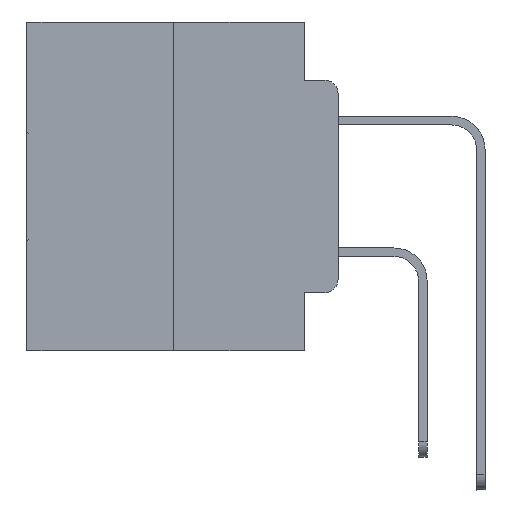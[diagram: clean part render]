
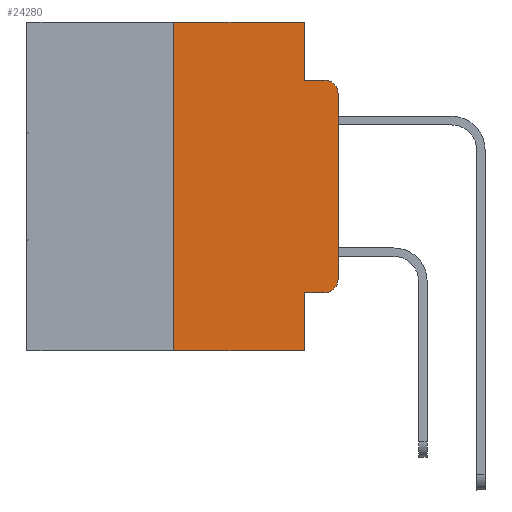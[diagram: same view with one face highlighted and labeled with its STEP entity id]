
A CAD part, left-side view. The second image highlights one B-rep face of the part: STEP entity #24280.
In plain terms, the highlighted planar face has unit normal (-1, 0, 0).
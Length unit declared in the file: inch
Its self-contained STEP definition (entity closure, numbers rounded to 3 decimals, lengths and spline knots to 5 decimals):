
#653 = EDGE_CURVE ( 'NONE', #25237, #11357, #2245, .T. ) ;
#929 = CARTESIAN_POINT ( 'NONE',  ( 0., 0.051, 0. ) ) ;
#1689 = VERTEX_POINT ( 'NONE', #3269 ) ;
#2054 = LINE ( 'NONE', #929, #7876 ) ;
#2245 = LINE ( 'NONE', #30359, #20890 ) ;
#2469 = VECTOR ( 'NONE', #9802, 39.37008 ) ;
#2824 = EDGE_CURVE ( 'NONE', #22098, #25548, #9690, .T. ) ;
#3015 = CARTESIAN_POINT ( 'NONE',  ( 0., 0., -0.3915 ) ) ;
#3049 = CARTESIAN_POINT ( 'NONE',  ( 0., 0., 0. ) ) ;
#3269 = CARTESIAN_POINT ( 'NONE',  ( 0., 0.02, -0.0885 ) ) ;
#3486 = DIRECTION ( 'NONE',  ( 0., 0., -1. ) ) ;
#3506 = AXIS2_PLACEMENT_3D ( 'NONE', #13708, #28260, #13824 ) ;
#3591 = CARTESIAN_POINT ( 'NONE',  ( 0., 0.25, 0. ) ) ;
#3608 = ORIENTED_EDGE ( 'NONE', *, *, #12410, .T. ) ;
#4257 = CARTESIAN_POINT ( 'NONE',  ( 0., 0.02, -0.1085 ) ) ;
#4287 = VERTEX_POINT ( 'NONE', #7870 ) ;
#4773 = VECTOR ( 'NONE', #27959, 39.37008 ) ;
#4962 = EDGE_LOOP ( 'NONE', ( #18984, #26924, #22753, #6592, #11934, #27152, #8615, #22231, #3608, #29385 ) ) ;
#6106 = DIRECTION ( 'NONE',  ( 0., 0., 1. ) ) ;
#6131 = VERTEX_POINT ( 'NONE', #3015 ) ;
#6236 = CARTESIAN_POINT ( 'NONE',  ( 0., 0.051, -0.0885 ) ) ;
#6496 = PLANE ( 'NONE',  #3506 ) ;
#6554 = FACE_OUTER_BOUND ( 'NONE', #4962, .T. ) ;
#6592 = ORIENTED_EDGE ( 'NONE', *, *, #20519, .F. ) ;
#6742 = DIRECTION ( 'NONE',  ( 0., 0., -1. ) ) ;
#7367 = CARTESIAN_POINT ( 'NONE',  ( 0., 0.051, 0. ) ) ;
#7427 = VECTOR ( 'NONE', #26977, 39.37008 ) ;
#7870 = CARTESIAN_POINT ( 'NONE',  ( 0., 0.051, -0.4115 ) ) ;
#7876 = VECTOR ( 'NONE', #3486, 39.37008 ) ;
#8458 = DIRECTION ( 'NONE',  ( -1., 0., 0. ) ) ;
#8495 = CARTESIAN_POINT ( 'NONE',  ( 0., 0., -0.1085 ) ) ;
#8614 = CARTESIAN_POINT ( 'NONE',  ( 0., 0.051, -0.0885 ) ) ;
#8615 = ORIENTED_EDGE ( 'NONE', *, *, #653, .T. ) ;
#9690 = LINE ( 'NONE', #19815, #21775 ) ;
#9732 = CARTESIAN_POINT ( 'NONE',  ( 0., 0.25, 0. ) ) ;
#9802 = DIRECTION ( 'NONE',  ( 0., 0., -1. ) ) ;
#10788 = EDGE_CURVE ( 'NONE', #22335, #6131, #20766, .T. ) ;
#11357 = VERTEX_POINT ( 'NONE', #15563 ) ;
#11416 = LINE ( 'NONE', #3049, #17154 ) ;
#11619 = LINE ( 'NONE', #7367, #2469 ) ;
#11934 = ORIENTED_EDGE ( 'NONE', *, *, #2824, .F. ) ;
#12024 = VERTEX_POINT ( 'NONE', #8495 ) ;
#12410 = EDGE_CURVE ( 'NONE', #4287, #22335, #13913, .T. ) ;
#13522 = VERTEX_POINT ( 'NONE', #6236 ) ;
#13708 = CARTESIAN_POINT ( 'NONE',  ( 0., 0.473, 0. ) ) ;
#13824 = DIRECTION ( 'NONE',  ( 0., 0., -1. ) ) ;
#13830 = CARTESIAN_POINT ( 'NONE',  ( 0., 0.25, -0.5 ) ) ;
#13913 = LINE ( 'NONE', #19788, #7427 ) ;
#14087 = AXIS2_PLACEMENT_3D ( 'NONE', #4257, #21222, #6742 ) ;
#15563 = CARTESIAN_POINT ( 'NONE',  ( 0., 0.051, -0.5 ) ) ;
#16010 = AXIS2_PLACEMENT_3D ( 'NONE', #22927, #8458, #25363 ) ;
#17154 = VECTOR ( 'NONE', #20070, 39.37008 ) ;
#17351 = EDGE_CURVE ( 'NONE', #4287, #11357, #11619, .T. ) ;
#18924 = EDGE_CURVE ( 'NONE', #25237, #22098, #21381, .T. ) ;
#18984 = ORIENTED_EDGE ( 'NONE', *, *, #30165, .T. ) ;
#19788 = CARTESIAN_POINT ( 'NONE',  ( 0., 0.051, -0.4115 ) ) ;
#19815 = CARTESIAN_POINT ( 'NONE',  ( 0., 0.473, 0. ) ) ;
#19908 = DIRECTION ( 'NONE',  ( 0., -1., 0. ) ) ;
#20070 = DIRECTION ( 'NONE',  ( 0., 0., 1. ) ) ;
#20519 = EDGE_CURVE ( 'NONE', #25548, #13522, #2054, .T. ) ;
#20525 = DIRECTION ( 'NONE',  ( 0., -1., 0. ) ) ;
#20766 = CIRCLE ( 'NONE', #16010, 0.02 ) ;
#20890 = VECTOR ( 'NONE', #20525, 39.37008 ) ;
#21222 = DIRECTION ( 'NONE',  ( -1., 0., 0. ) ) ;
#21357 = CIRCLE ( 'NONE', #14087, 0.02 ) ;
#21381 = LINE ( 'NONE', #3591, #27822 ) ;
#21775 = VECTOR ( 'NONE', #19908, 39.37008 ) ;
#22098 = VERTEX_POINT ( 'NONE', #9732 ) ;
#22111 = CARTESIAN_POINT ( 'NONE',  ( 0., 0.051, 0. ) ) ;
#22231 = ORIENTED_EDGE ( 'NONE', *, *, #17351, .F. ) ;
#22335 = VERTEX_POINT ( 'NONE', #30088 ) ;
#22753 = ORIENTED_EDGE ( 'NONE', *, *, #27018, .F. ) ;
#22927 = CARTESIAN_POINT ( 'NONE',  ( 0., 0.02, -0.3915 ) ) ;
#24280 = ADVANCED_FACE ( 'NONE', ( #6554 ), #6496, .F. ) ;
#24895 = LINE ( 'NONE', #8614, #4773 ) ;
#25237 = VERTEX_POINT ( 'NONE', #13830 ) ;
#25363 = DIRECTION ( 'NONE',  ( 0., 0., -1. ) ) ;
#25548 = VERTEX_POINT ( 'NONE', #22111 ) ;
#26924 = ORIENTED_EDGE ( 'NONE', *, *, #28608, .T. ) ;
#26977 = DIRECTION ( 'NONE',  ( 0., -1., 0. ) ) ;
#27018 = EDGE_CURVE ( 'NONE', #13522, #1689, #24895, .T. ) ;
#27152 = ORIENTED_EDGE ( 'NONE', *, *, #18924, .F. ) ;
#27822 = VECTOR ( 'NONE', #6106, 39.37008 ) ;
#27959 = DIRECTION ( 'NONE',  ( 0., -1., 0. ) ) ;
#28260 = DIRECTION ( 'NONE',  ( 1., 0., 0. ) ) ;
#28608 = EDGE_CURVE ( 'NONE', #12024, #1689, #21357, .T. ) ;
#29385 = ORIENTED_EDGE ( 'NONE', *, *, #10788, .T. ) ;
#30088 = CARTESIAN_POINT ( 'NONE',  ( 0., 0.02, -0.4115 ) ) ;
#30165 = EDGE_CURVE ( 'NONE', #6131, #12024, #11416, .T. ) ;
#30359 = CARTESIAN_POINT ( 'NONE',  ( 0., 0.473, -0.5 ) ) ;
